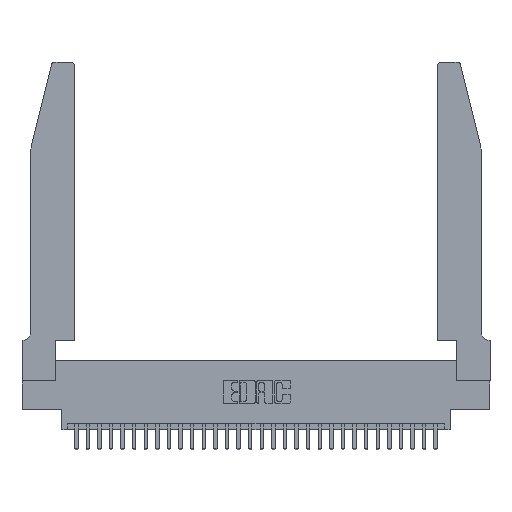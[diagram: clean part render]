
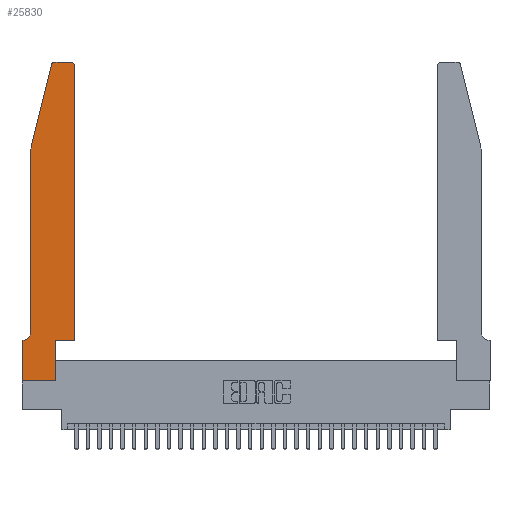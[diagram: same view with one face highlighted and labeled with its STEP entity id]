
A CAD part, top view. The second image highlights one B-rep face of the part: STEP entity #25830.
In plain terms, the highlighted planar face has unit normal (0, 0, 1).
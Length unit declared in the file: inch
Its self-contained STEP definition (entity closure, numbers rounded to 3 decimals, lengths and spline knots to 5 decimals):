
#18 = ORIENTED_EDGE ( 'NONE', *, *, #27743, .T. ) ;
#709 = AXIS2_PLACEMENT_3D ( 'NONE', #12882, #29785, #15281 ) ;
#941 = ORIENTED_EDGE ( 'NONE', *, *, #5154, .T. ) ;
#1314 = VECTOR ( 'NONE', #26437, 39.37008 ) ;
#1836 = LINE ( 'NONE', #31085, #20531 ) ;
#1962 = VECTOR ( 'NONE', #20172, 39.37008 ) ;
#2122 = LINE ( 'NONE', #28630, #14349 ) ;
#2511 = LINE ( 'NONE', #11040, #13999 ) ;
#2541 = VERTEX_POINT ( 'NONE', #11604 ) ;
#2894 = FACE_OUTER_BOUND ( 'NONE', #12789, .T. ) ;
#3733 = CARTESIAN_POINT ( 'NONE',  ( 0.0755, 2., 0.37 ) ) ;
#4022 = CARTESIAN_POINT ( 'NONE',  ( 0.0755, 0.35, 0.37 ) ) ;
#4047 = LINE ( 'NONE', #8125, #9839 ) ;
#4425 = DIRECTION ( 'NONE',  ( 0., -1., 0. ) ) ;
#4562 = EDGE_CURVE ( 'NONE', #7611, #2541, #4047, .T. ) ;
#4878 = CARTESIAN_POINT ( 'NONE',  ( 0.2865, 0.35, 0.37 ) ) ;
#5154 = EDGE_CURVE ( 'NONE', #20971, #16345, #21193, .T. ) ;
#5569 = CARTESIAN_POINT ( 'NONE',  ( 0.0755, 0.42, 0.37 ) ) ;
#5863 = CARTESIAN_POINT ( 'NONE',  ( 0.0055, 0.35, 0.37 ) ) ;
#6307 = ORIENTED_EDGE ( 'NONE', *, *, #8970, .T. ) ;
#7077 = EDGE_CURVE ( 'NONE', #14719, #25573, #29371, .T. ) ;
#7611 = VERTEX_POINT ( 'NONE', #15684 ) ;
#8125 = CARTESIAN_POINT ( 'NONE',  ( 0., 0., 0.37 ) ) ;
#8360 = CARTESIAN_POINT ( 'NONE',  ( 0.4505, 0.35, 0.37 ) ) ;
#8681 = ORIENTED_EDGE ( 'NONE', *, *, #23981, .T. ) ;
#8970 = EDGE_CURVE ( 'NONE', #14015, #20971, #24801, .T. ) ;
#9303 = VERTEX_POINT ( 'NONE', #19204 ) ;
#9484 = CARTESIAN_POINT ( 'NONE',  ( 0.2605, 2.75, 0.37 ) ) ;
#9839 = VECTOR ( 'NONE', #10594, 39.37008 ) ;
#10424 = AXIS2_PLACEMENT_3D ( 'NONE', #18508, #11425, #28338 ) ;
#10532 = ORIENTED_EDGE ( 'NONE', *, *, #11829, .T. ) ;
#10594 = DIRECTION ( 'NONE',  ( 1., 0., 0. ) ) ;
#11040 = CARTESIAN_POINT ( 'NONE',  ( 0.4505, 0.35, 0.37 ) ) ;
#11425 = DIRECTION ( 'NONE',  ( 0., 0., 1. ) ) ;
#11604 = CARTESIAN_POINT ( 'NONE',  ( 0.2865, 0., 0.37 ) ) ;
#11829 = EDGE_CURVE ( 'NONE', #2541, #18427, #2122, .T. ) ;
#12594 = ORIENTED_EDGE ( 'NONE', *, *, #26014, .T. ) ;
#12789 = EDGE_LOOP ( 'NONE', ( #17154, #15588, #23458, #6307, #941, #28872, #8681, #18696, #10532, #18, #24594, #12594 ) ) ;
#12882 = CARTESIAN_POINT ( 'NONE',  ( 0.0055, 0.42, 0.37 ) ) ;
#12966 = EDGE_CURVE ( 'NONE', #16345, #9303, #16951, .T. ) ;
#13198 = DIRECTION ( 'NONE',  ( 0., 0., 1. ) ) ;
#13999 = VECTOR ( 'NONE', #30388, 39.37008 ) ;
#14015 = VERTEX_POINT ( 'NONE', #3733 ) ;
#14299 = LINE ( 'NONE', #9484, #1314 ) ;
#14349 = VECTOR ( 'NONE', #31065, 39.37008 ) ;
#14537 = CARTESIAN_POINT ( 'NONE',  ( 0.4205, 2.72, 0.37 ) ) ;
#14719 = VERTEX_POINT ( 'NONE', #28880 ) ;
#15281 = DIRECTION ( 'NONE',  ( -1., 0., 0. ) ) ;
#15588 = ORIENTED_EDGE ( 'NONE', *, *, #7077, .T. ) ;
#15684 = CARTESIAN_POINT ( 'NONE',  ( 0., 0., 0.37 ) ) ;
#16167 = PLANE ( 'NONE',  #10424 ) ;
#16188 = VECTOR ( 'NONE', #25950, 39.37008 ) ;
#16345 = VERTEX_POINT ( 'NONE', #5863 ) ;
#16951 = LINE ( 'NONE', #4022, #16188 ) ;
#16998 = DIRECTION ( 'NONE',  ( 1., 0., 0. ) ) ;
#17154 = ORIENTED_EDGE ( 'NONE', *, *, #29573, .T. ) ;
#17446 = VERTEX_POINT ( 'NONE', #27652 ) ;
#17607 = CARTESIAN_POINT ( 'NONE',  ( 0.0755, 2., 0.37 ) ) ;
#18427 = VERTEX_POINT ( 'NONE', #4878 ) ;
#18508 = CARTESIAN_POINT ( 'NONE',  ( 0., 0.35, 0.37 ) ) ;
#18696 = ORIENTED_EDGE ( 'NONE', *, *, #4562, .T. ) ;
#19204 = CARTESIAN_POINT ( 'NONE',  ( 0., 0.35, 0.37 ) ) ;
#20172 = DIRECTION ( 'NONE',  ( -0.239, -0.971, 0. ) ) ;
#20531 = VECTOR ( 'NONE', #4425, 39.37008 ) ;
#20971 = VERTEX_POINT ( 'NONE', #5569 ) ;
#21193 = CIRCLE ( 'NONE', #709, 0.07 ) ;
#22559 = CARTESIAN_POINT ( 'NONE',  ( 0.25487, 2.72718, 0.37 ) ) ;
#22917 = DIRECTION ( 'NONE',  ( 0., 1., 0. ) ) ;
#23458 = ORIENTED_EDGE ( 'NONE', *, *, #31413, .T. ) ;
#23513 = CIRCLE ( 'NONE', #28270, 0.03 ) ;
#23981 = EDGE_CURVE ( 'NONE', #9303, #7611, #1836, .T. ) ;
#24255 = VERTEX_POINT ( 'NONE', #24745 ) ;
#24594 = ORIENTED_EDGE ( 'NONE', *, *, #25040, .T. ) ;
#24745 = CARTESIAN_POINT ( 'NONE',  ( 0.4505, 2.72, 0.37 ) ) ;
#24801 = LINE ( 'NONE', #27752, #29673 ) ;
#25040 = EDGE_CURVE ( 'NONE', #28271, #24255, #26581, .T. ) ;
#25412 = CARTESIAN_POINT ( 'NONE',  ( 0.4505, 0.35, 0.37 ) ) ;
#25431 = AXIS2_PLACEMENT_3D ( 'NONE', #27691, #13198, #30127 ) ;
#25573 = VERTEX_POINT ( 'NONE', #22559 ) ;
#25830 = ADVANCED_FACE ( 'NONE', ( #2894 ), #16167, .T. ) ;
#25950 = DIRECTION ( 'NONE',  ( -1., 0., 0. ) ) ;
#26014 = EDGE_CURVE ( 'NONE', #24255, #17446, #23513, .T. ) ;
#26360 = DIRECTION ( 'NONE',  ( 0., 0., 1. ) ) ;
#26437 = DIRECTION ( 'NONE',  ( -1., 0., 0. ) ) ;
#26581 = LINE ( 'NONE', #8360, #29944 ) ;
#27652 = CARTESIAN_POINT ( 'NONE',  ( 0.4205, 2.75, 0.37 ) ) ;
#27691 = CARTESIAN_POINT ( 'NONE',  ( 0.284, 2.72, 0.37 ) ) ;
#27743 = EDGE_CURVE ( 'NONE', #18427, #28271, #2511, .T. ) ;
#27752 = CARTESIAN_POINT ( 'NONE',  ( 0.0755, 2., 0.37 ) ) ;
#28270 = AXIS2_PLACEMENT_3D ( 'NONE', #14537, #26360, #16998 ) ;
#28271 = VERTEX_POINT ( 'NONE', #25412 ) ;
#28338 = DIRECTION ( 'NONE',  ( 1., 0., 0. ) ) ;
#28589 = LINE ( 'NONE', #17607, #1962 ) ;
#28630 = CARTESIAN_POINT ( 'NONE',  ( 0.2865, 0.35, 0.37 ) ) ;
#28872 = ORIENTED_EDGE ( 'NONE', *, *, #12966, .T. ) ;
#28880 = CARTESIAN_POINT ( 'NONE',  ( 0.284, 2.75, 0.37 ) ) ;
#29371 = CIRCLE ( 'NONE', #25431, 0.03 ) ;
#29573 = EDGE_CURVE ( 'NONE', #17446, #14719, #14299, .T. ) ;
#29673 = VECTOR ( 'NONE', #30182, 39.37008 ) ;
#29785 = DIRECTION ( 'NONE',  ( 0., 0., -1. ) ) ;
#29944 = VECTOR ( 'NONE', #22917, 39.37008 ) ;
#30127 = DIRECTION ( 'NONE',  ( 1., 0., 0. ) ) ;
#30182 = DIRECTION ( 'NONE',  ( 0., -1., 0. ) ) ;
#30388 = DIRECTION ( 'NONE',  ( 1., 0., 0. ) ) ;
#31065 = DIRECTION ( 'NONE',  ( 0., 1., 0. ) ) ;
#31085 = CARTESIAN_POINT ( 'NONE',  ( 0., 0., 0.37 ) ) ;
#31413 = EDGE_CURVE ( 'NONE', #25573, #14015, #28589, .T. ) ;
